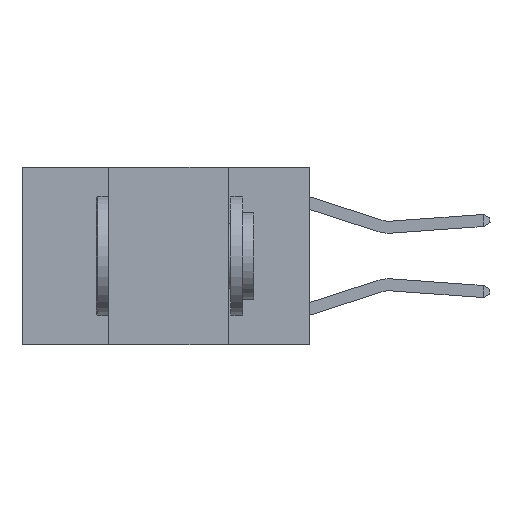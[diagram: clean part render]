
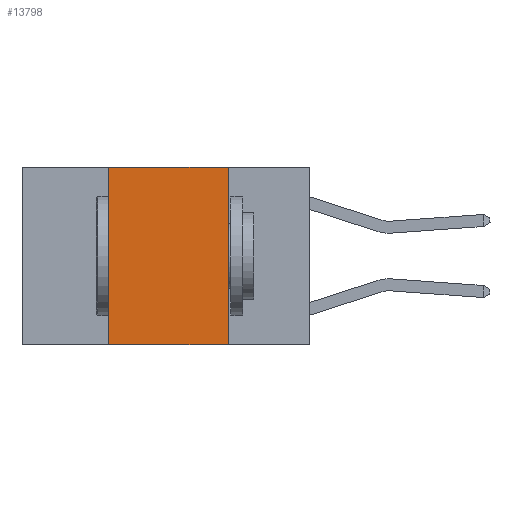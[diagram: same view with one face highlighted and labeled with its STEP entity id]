
A CAD part, left-side view. The second image highlights one B-rep face of the part: STEP entity #13798.
In plain terms, the highlighted planar face has unit normal (-1, 0, 0).
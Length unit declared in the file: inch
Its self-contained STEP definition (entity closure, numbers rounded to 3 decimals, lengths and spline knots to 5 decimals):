
#1659 = CARTESIAN_POINT ( 'NONE',  ( 0., 0.17, 0. ) ) ;
#2235 = DIRECTION ( 'NONE',  ( 0., 0., -1. ) ) ;
#4394 = ORIENTED_EDGE ( 'NONE', *, *, #13087, .T. ) ;
#4529 = CARTESIAN_POINT ( 'NONE',  ( 0., 0.6, 0. ) ) ;
#4750 = LINE ( 'NONE', #14287, #15261 ) ;
#4982 = CARTESIAN_POINT ( 'NONE',  ( 0., 0.6, 0. ) ) ;
#5120 = ORIENTED_EDGE ( 'NONE', *, *, #12759, .F. ) ;
#5344 = FACE_OUTER_BOUND ( 'NONE', #15135, .T. ) ;
#5848 = CARTESIAN_POINT ( 'NONE',  ( 0., 0.42, -0.37 ) ) ;
#6802 = VERTEX_POINT ( 'NONE', #14892 ) ;
#7182 = EDGE_CURVE ( 'NONE', #16797, #9110, #4750, .T. ) ;
#7415 = CARTESIAN_POINT ( 'NONE',  ( 0., 0.42, 0. ) ) ;
#8724 = DIRECTION ( 'NONE',  ( 0., 0., -1. ) ) ;
#8925 = ORIENTED_EDGE ( 'NONE', *, *, #7182, .F. ) ;
#9110 = VERTEX_POINT ( 'NONE', #7415 ) ;
#11633 = DIRECTION ( 'NONE',  ( 0., 0., 1. ) ) ;
#11946 = CARTESIAN_POINT ( 'NONE',  ( 0., 0.17, 0. ) ) ;
#12225 = LINE ( 'NONE', #14157, #15415 ) ;
#12757 = AXIS2_PLACEMENT_3D ( 'NONE', #4529, #16877, #8724 ) ;
#12759 = EDGE_CURVE ( 'NONE', #9110, #15035, #16476, .T. ) ;
#12776 = PLANE ( 'NONE',  #12757 ) ;
#13087 = EDGE_CURVE ( 'NONE', #16797, #6802, #12225, .T. ) ;
#13210 = DIRECTION ( 'NONE',  ( 0., -1., 0. ) ) ;
#13798 = ADVANCED_FACE ( 'NONE', ( #5344 ), #12776, .F. ) ;
#14157 = CARTESIAN_POINT ( 'NONE',  ( 0., 0.6, -0.37 ) ) ;
#14277 = LINE ( 'NONE', #11946, #16607 ) ;
#14287 = CARTESIAN_POINT ( 'NONE',  ( 0., 0.42, 0. ) ) ;
#14892 = CARTESIAN_POINT ( 'NONE',  ( 0., 0.17, -0.37 ) ) ;
#15035 = VERTEX_POINT ( 'NONE', #1659 ) ;
#15135 = EDGE_LOOP ( 'NONE', ( #16202, #5120, #8925, #4394 ) ) ;
#15261 = VECTOR ( 'NONE', #11633, 39.37008 ) ;
#15415 = VECTOR ( 'NONE', #15536, 39.37008 ) ;
#15536 = DIRECTION ( 'NONE',  ( 0., -1., 0. ) ) ;
#16202 = ORIENTED_EDGE ( 'NONE', *, *, #16340, .F. ) ;
#16340 = EDGE_CURVE ( 'NONE', #15035, #6802, #14277, .T. ) ;
#16476 = LINE ( 'NONE', #4982, #16913 ) ;
#16607 = VECTOR ( 'NONE', #2235, 39.37008 ) ;
#16797 = VERTEX_POINT ( 'NONE', #5848 ) ;
#16877 = DIRECTION ( 'NONE',  ( 1., 0., 0. ) ) ;
#16913 = VECTOR ( 'NONE', #13210, 39.37008 ) ;
